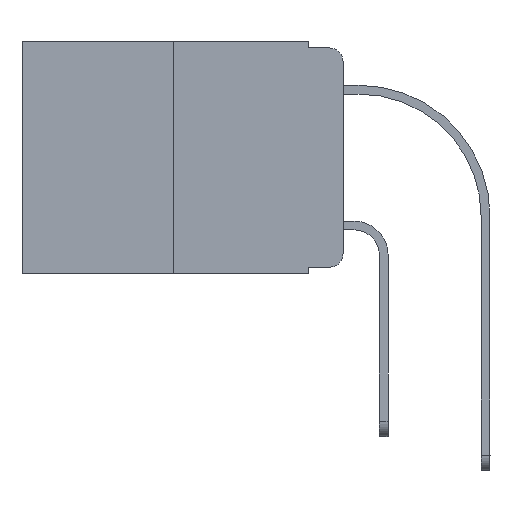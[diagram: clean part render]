
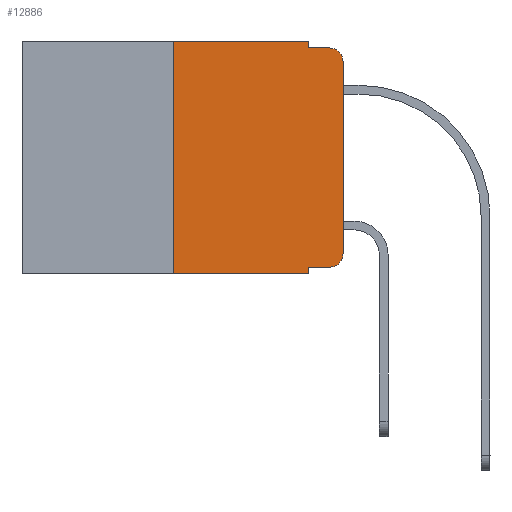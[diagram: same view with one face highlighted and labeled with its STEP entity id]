
A CAD part, left-side view. The second image highlights one B-rep face of the part: STEP entity #12886.
In plain terms, the highlighted planar face has unit normal (-1, 0, 0).
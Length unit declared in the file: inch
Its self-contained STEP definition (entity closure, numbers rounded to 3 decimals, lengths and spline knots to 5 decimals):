
#58 = DIRECTION ( 'NONE',  ( 0., 0., -1. ) ) ;
#822 = LINE ( 'NONE', #12280, #4019 ) ;
#981 = CARTESIAN_POINT ( 'NONE',  ( 0., 0.25, -0.343 ) ) ;
#997 = ORIENTED_EDGE ( 'NONE', *, *, #9636, .T. ) ;
#1148 = VERTEX_POINT ( 'NONE', #13200 ) ;
#1493 = VERTEX_POINT ( 'NONE', #15846 ) ;
#1516 = CARTESIAN_POINT ( 'NONE',  ( 0., 0.473, 0. ) ) ;
#1586 = VECTOR ( 'NONE', #58, 39.37008 ) ;
#2402 = EDGE_CURVE ( 'NONE', #19009, #1493, #21195, .T. ) ;
#2473 = DIRECTION ( 'NONE',  ( 0., -1., 0. ) ) ;
#2743 = ORIENTED_EDGE ( 'NONE', *, *, #3574, .T. ) ;
#2988 = CIRCLE ( 'NONE', #21138, 0.02 ) ;
#3275 = DIRECTION ( 'NONE',  ( 0., -1., 0. ) ) ;
#3474 = ORIENTED_EDGE ( 'NONE', *, *, #11691, .F. ) ;
#3506 = CARTESIAN_POINT ( 'NONE',  ( 0., 0.051, -0.333 ) ) ;
#3574 = EDGE_CURVE ( 'NONE', #19009, #4306, #19690, .T. ) ;
#3667 = DIRECTION ( 'NONE',  ( 0., 0., -1. ) ) ;
#3928 = VERTEX_POINT ( 'NONE', #16918 ) ;
#4004 = EDGE_CURVE ( 'NONE', #9463, #1493, #10203, .T. ) ;
#4019 = VECTOR ( 'NONE', #14082, 39.37008 ) ;
#4121 = ORIENTED_EDGE ( 'NONE', *, *, #12245, .F. ) ;
#4306 = VERTEX_POINT ( 'NONE', #8672 ) ;
#4495 = CARTESIAN_POINT ( 'NONE',  ( 0., 0.051, -0.333 ) ) ;
#5424 = LINE ( 'NONE', #13829, #9844 ) ;
#5873 = PLANE ( 'NONE',  #14097 ) ;
#6398 = EDGE_CURVE ( 'NONE', #17633, #6568, #9490, .T. ) ;
#6568 = VERTEX_POINT ( 'NONE', #20108 ) ;
#7630 = CARTESIAN_POINT ( 'NONE',  ( 0., 0.473, -0.343 ) ) ;
#8213 = CARTESIAN_POINT ( 'NONE',  ( 0., 0.051, -0.01 ) ) ;
#8621 = VERTEX_POINT ( 'NONE', #11734 ) ;
#8672 = CARTESIAN_POINT ( 'NONE',  ( 0., 0.02, -0.333 ) ) ;
#9447 = AXIS2_PLACEMENT_3D ( 'NONE', #13602, #14982, #3667 ) ;
#9463 = VERTEX_POINT ( 'NONE', #981 ) ;
#9490 = LINE ( 'NONE', #8213, #12333 ) ;
#9636 = EDGE_CURVE ( 'NONE', #13107, #6568, #2988, .T. ) ;
#9844 = VECTOR ( 'NONE', #20408, 39.37008 ) ;
#10131 = CARTESIAN_POINT ( 'NONE',  ( 0., 0.051, 0. ) ) ;
#10203 = LINE ( 'NONE', #7630, #14981 ) ;
#10376 = CARTESIAN_POINT ( 'NONE',  ( 0., 0.051, -0.01 ) ) ;
#10434 = ORIENTED_EDGE ( 'NONE', *, *, #18449, .T. ) ;
#10577 = CARTESIAN_POINT ( 'NONE',  ( 0., 0.473, 0. ) ) ;
#11272 = LINE ( 'NONE', #1516, #13579 ) ;
#11691 = EDGE_CURVE ( 'NONE', #9463, #8621, #822, .T. ) ;
#11734 = CARTESIAN_POINT ( 'NONE',  ( 0., 0.25, 0. ) ) ;
#11925 = VECTOR ( 'NONE', #16442, 39.37008 ) ;
#11965 = DIRECTION ( 'NONE',  ( 1., 0., 0. ) ) ;
#12011 = EDGE_CURVE ( 'NONE', #1148, #13107, #5424, .T. ) ;
#12245 = EDGE_CURVE ( 'NONE', #8621, #3928, #11272, .T. ) ;
#12280 = CARTESIAN_POINT ( 'NONE',  ( 0., 0.25, 0. ) ) ;
#12333 = VECTOR ( 'NONE', #3275, 39.37008 ) ;
#12500 = CIRCLE ( 'NONE', #9447, 0.02 ) ;
#12886 = ADVANCED_FACE ( 'NONE', ( #20655 ), #5873, .F. ) ;
#13107 = VERTEX_POINT ( 'NONE', #14903 ) ;
#13200 = CARTESIAN_POINT ( 'NONE',  ( 0., 0., -0.313 ) ) ;
#13336 = EDGE_LOOP ( 'NONE', ( #17802, #997, #20428, #20984, #4121, #3474, #17549, #19996, #2743, #10434 ) ) ;
#13579 = VECTOR ( 'NONE', #17818, 39.37008 ) ;
#13602 = CARTESIAN_POINT ( 'NONE',  ( 0., 0.02, -0.313 ) ) ;
#13829 = CARTESIAN_POINT ( 'NONE',  ( 0., 0., 0. ) ) ;
#14082 = DIRECTION ( 'NONE',  ( 0., 0., 1. ) ) ;
#14097 = AXIS2_PLACEMENT_3D ( 'NONE', #10577, #11965, #17091 ) ;
#14604 = DIRECTION ( 'NONE',  ( 0., 0., -1. ) ) ;
#14903 = CARTESIAN_POINT ( 'NONE',  ( 0., 0., -0.03 ) ) ;
#14981 = VECTOR ( 'NONE', #2473, 39.37008 ) ;
#14982 = DIRECTION ( 'NONE',  ( -1., 0., 0. ) ) ;
#15846 = CARTESIAN_POINT ( 'NONE',  ( 0., 0.051, -0.343 ) ) ;
#16155 = DIRECTION ( 'NONE',  ( -1., 0., 0. ) ) ;
#16442 = DIRECTION ( 'NONE',  ( 0., -1., 0. ) ) ;
#16570 = VECTOR ( 'NONE', #14604, 39.37008 ) ;
#16918 = CARTESIAN_POINT ( 'NONE',  ( 0., 0.051, 0. ) ) ;
#17091 = DIRECTION ( 'NONE',  ( 0., 0., -1. ) ) ;
#17549 = ORIENTED_EDGE ( 'NONE', *, *, #4004, .T. ) ;
#17633 = VERTEX_POINT ( 'NONE', #10376 ) ;
#17690 = CARTESIAN_POINT ( 'NONE',  ( 0., 0.02, -0.03 ) ) ;
#17802 = ORIENTED_EDGE ( 'NONE', *, *, #12011, .T. ) ;
#17804 = DIRECTION ( 'NONE',  ( 0., 0., -1. ) ) ;
#17818 = DIRECTION ( 'NONE',  ( 0., -1., 0. ) ) ;
#17854 = LINE ( 'NONE', #10131, #16570 ) ;
#18449 = EDGE_CURVE ( 'NONE', #4306, #1148, #12500, .T. ) ;
#19009 = VERTEX_POINT ( 'NONE', #4495 ) ;
#19689 = CARTESIAN_POINT ( 'NONE',  ( 0., 0.051, 0. ) ) ;
#19690 = LINE ( 'NONE', #3506, #11925 ) ;
#19996 = ORIENTED_EDGE ( 'NONE', *, *, #2402, .F. ) ;
#20108 = CARTESIAN_POINT ( 'NONE',  ( 0., 0.02, -0.01 ) ) ;
#20408 = DIRECTION ( 'NONE',  ( 0., 0., 1. ) ) ;
#20428 = ORIENTED_EDGE ( 'NONE', *, *, #6398, .F. ) ;
#20642 = EDGE_CURVE ( 'NONE', #3928, #17633, #17854, .T. ) ;
#20655 = FACE_OUTER_BOUND ( 'NONE', #13336, .T. ) ;
#20984 = ORIENTED_EDGE ( 'NONE', *, *, #20642, .F. ) ;
#21138 = AXIS2_PLACEMENT_3D ( 'NONE', #17690, #16155, #17804 ) ;
#21195 = LINE ( 'NONE', #19689, #1586 ) ;
